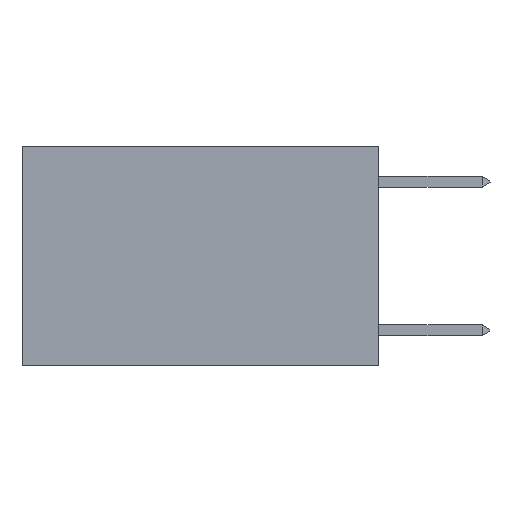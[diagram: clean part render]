
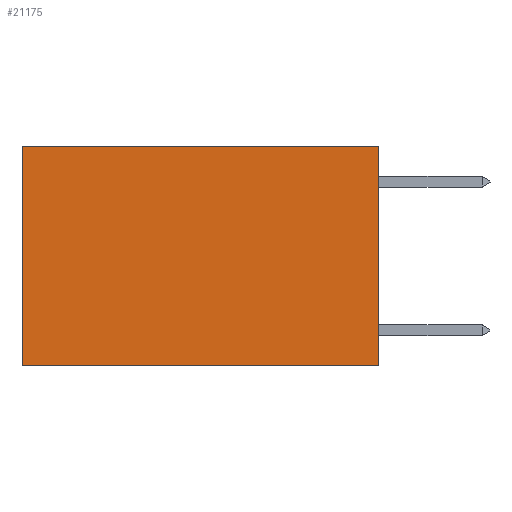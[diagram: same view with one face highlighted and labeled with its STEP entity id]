
A CAD part, left-side view. The second image highlights one B-rep face of the part: STEP entity #21175.
In plain terms, the highlighted planar face has unit normal (-1, 0, 0).
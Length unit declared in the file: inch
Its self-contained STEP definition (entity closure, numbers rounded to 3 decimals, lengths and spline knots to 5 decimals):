
#705 = CARTESIAN_POINT ( 'NONE',  ( 0.2625, 0., 0. ) ) ;
#829 = CARTESIAN_POINT ( 'NONE',  ( 0.2625, 0.6, 0. ) ) ;
#1880 = AXIS2_PLACEMENT_3D ( 'NONE', #21160, #7329, #9332 ) ;
#2622 = DIRECTION ( 'NONE',  ( 0., 1., 0. ) ) ;
#2881 = VERTEX_POINT ( 'NONE', #17669 ) ;
#3170 = CARTESIAN_POINT ( 'NONE',  ( 0.2625, 0., 0. ) ) ;
#3400 = VECTOR ( 'NONE', #7238, 39.37008 ) ;
#3735 = ORIENTED_EDGE ( 'NONE', *, *, #21581, .F. ) ;
#4909 = FACE_OUTER_BOUND ( 'NONE', #17821, .T. ) ;
#5331 = VECTOR ( 'NONE', #2622, 39.37008 ) ;
#5515 = CARTESIAN_POINT ( 'NONE',  ( 0.2625, 0., 0. ) ) ;
#5691 = ORIENTED_EDGE ( 'NONE', *, *, #11913, .T. ) ;
#6491 = VECTOR ( 'NONE', #6712, 39.37008 ) ;
#6634 = VECTOR ( 'NONE', #8635, 39.37008 ) ;
#6712 = DIRECTION ( 'NONE',  ( 0., 1., 0. ) ) ;
#7238 = DIRECTION ( 'NONE',  ( 0., 0., -1. ) ) ;
#7329 = DIRECTION ( 'NONE',  ( 1., 0., 0. ) ) ;
#7776 = VERTEX_POINT ( 'NONE', #18098 ) ;
#8635 = DIRECTION ( 'NONE',  ( 0., 0., -1. ) ) ;
#9332 = DIRECTION ( 'NONE',  ( 0., 0., -1. ) ) ;
#10197 = LINE ( 'NONE', #705, #6491 ) ;
#11093 = CARTESIAN_POINT ( 'NONE',  ( 0.2625, 0.6, 0. ) ) ;
#11591 = ORIENTED_EDGE ( 'NONE', *, *, #15894, .T. ) ;
#11913 = EDGE_CURVE ( 'NONE', #17500, #2881, #22461, .T. ) ;
#12733 = ORIENTED_EDGE ( 'NONE', *, *, #23385, .F. ) ;
#14514 = CARTESIAN_POINT ( 'NONE',  ( 0.2625, 0., -0.37 ) ) ;
#14843 = VERTEX_POINT ( 'NONE', #3170 ) ;
#15894 = EDGE_CURVE ( 'NONE', #14843, #17500, #10197, .T. ) ;
#17500 = VERTEX_POINT ( 'NONE', #11093 ) ;
#17669 = CARTESIAN_POINT ( 'NONE',  ( 0.2625, 0.6, -0.37 ) ) ;
#17821 = EDGE_LOOP ( 'NONE', ( #5691, #3735, #12733, #11591 ) ) ;
#18098 = CARTESIAN_POINT ( 'NONE',  ( 0.2625, 0., -0.37 ) ) ;
#19274 = PLANE ( 'NONE',  #1880 ) ;
#21160 = CARTESIAN_POINT ( 'NONE',  ( 0.2625, 0., 0. ) ) ;
#21175 = ADVANCED_FACE ( 'NONE', ( #4909 ), #19274, .F. ) ;
#21468 = LINE ( 'NONE', #14514, #5331 ) ;
#21581 = EDGE_CURVE ( 'NONE', #7776, #2881, #21468, .T. ) ;
#22461 = LINE ( 'NONE', #829, #6634 ) ;
#23385 = EDGE_CURVE ( 'NONE', #14843, #7776, #23562, .T. ) ;
#23562 = LINE ( 'NONE', #5515, #3400 ) ;
